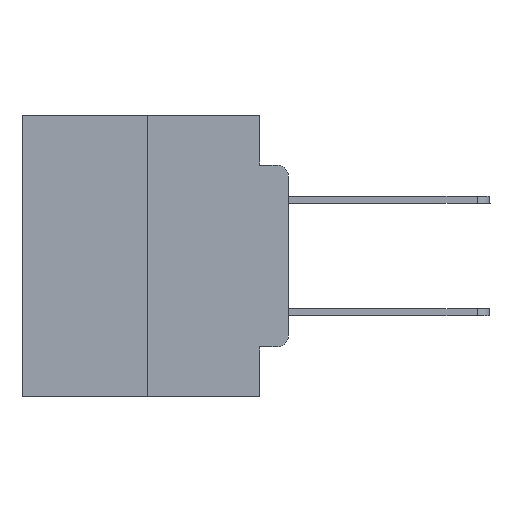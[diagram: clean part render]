
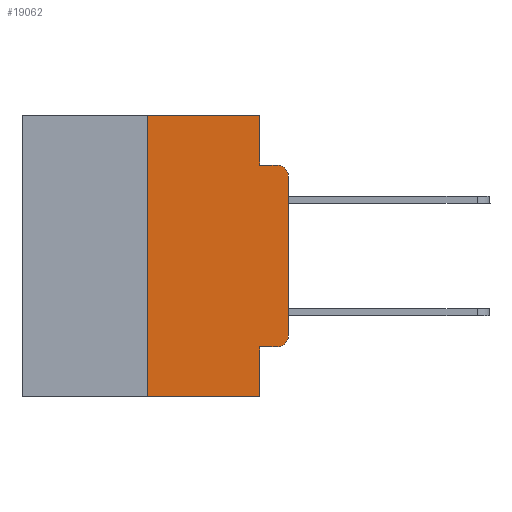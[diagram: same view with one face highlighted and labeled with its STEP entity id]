
A CAD part, left-side view. The second image highlights one B-rep face of the part: STEP entity #19062.
In plain terms, the highlighted planar face has unit normal (-1, 0, 0).
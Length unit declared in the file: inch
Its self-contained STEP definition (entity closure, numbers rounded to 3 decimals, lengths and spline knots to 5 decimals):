
#301 = DIRECTION ( 'NONE',  ( -1., 0., 0. ) ) ;
#646 = EDGE_CURVE ( 'NONE', #17560, #13822, #26466, .T. ) ;
#674 = VECTOR ( 'NONE', #2871, 39.37008 ) ;
#688 = CARTESIAN_POINT ( 'NONE',  ( 0., 0.051, 0. ) ) ;
#903 = CARTESIAN_POINT ( 'NONE',  ( 0., 0.051, -0.0885 ) ) ;
#1089 = VERTEX_POINT ( 'NONE', #4384 ) ;
#2356 = DIRECTION ( 'NONE',  ( 0., 0., -1. ) ) ;
#2700 = VERTEX_POINT ( 'NONE', #14157 ) ;
#2746 = ORIENTED_EDGE ( 'NONE', *, *, #14768, .T. ) ;
#2825 = DIRECTION ( 'NONE',  ( 0., 0., 1. ) ) ;
#2871 = DIRECTION ( 'NONE',  ( 0., -1., 0. ) ) ;
#2971 = EDGE_CURVE ( 'NONE', #7550, #22965, #7790, .T. ) ;
#3133 = EDGE_CURVE ( 'NONE', #5858, #2700, #3486, .T. ) ;
#3486 = CIRCLE ( 'NONE', #5319, 0.02 ) ;
#3711 = VECTOR ( 'NONE', #15448, 39.37008 ) ;
#4319 = VECTOR ( 'NONE', #15468, 39.37008 ) ;
#4364 = LINE ( 'NONE', #21749, #3711 ) ;
#4384 = CARTESIAN_POINT ( 'NONE',  ( 0., 0.051, -0.4115 ) ) ;
#4393 = CARTESIAN_POINT ( 'NONE',  ( 0., 0.02, -0.1085 ) ) ;
#4721 = VECTOR ( 'NONE', #10827, 39.37008 ) ;
#5225 = ORIENTED_EDGE ( 'NONE', *, *, #14411, .T. ) ;
#5319 = AXIS2_PLACEMENT_3D ( 'NONE', #8738, #301, #23548 ) ;
#5858 = VERTEX_POINT ( 'NONE', #16393 ) ;
#6036 = ORIENTED_EDGE ( 'NONE', *, *, #646, .F. ) ;
#6722 = LINE ( 'NONE', #23231, #4721 ) ;
#7337 = ORIENTED_EDGE ( 'NONE', *, *, #17486, .T. ) ;
#7550 = VERTEX_POINT ( 'NONE', #10167 ) ;
#7790 = CIRCLE ( 'NONE', #11848, 0.02 ) ;
#8301 = LINE ( 'NONE', #9455, #674 ) ;
#8578 = CARTESIAN_POINT ( 'NONE',  ( 0., 0.051, -0.5 ) ) ;
#8738 = CARTESIAN_POINT ( 'NONE',  ( 0., 0.02, -0.3915 ) ) ;
#8921 = EDGE_CURVE ( 'NONE', #1089, #23056, #6722, .T. ) ;
#9004 = CARTESIAN_POINT ( 'NONE',  ( 0., 0.051, 0. ) ) ;
#9455 = CARTESIAN_POINT ( 'NONE',  ( 0., 0.051, -0.4115 ) ) ;
#9891 = DIRECTION ( 'NONE',  ( 0., 0., -1. ) ) ;
#9920 = EDGE_CURVE ( 'NONE', #17055, #17560, #24547, .T. ) ;
#10167 = CARTESIAN_POINT ( 'NONE',  ( 0., 0., -0.1085 ) ) ;
#10489 = ORIENTED_EDGE ( 'NONE', *, *, #14326, .F. ) ;
#10553 = AXIS2_PLACEMENT_3D ( 'NONE', #26771, #22561, #9891 ) ;
#10827 = DIRECTION ( 'NONE',  ( 0., 0., -1. ) ) ;
#11048 = CARTESIAN_POINT ( 'NONE',  ( 0., 0.25, -0.5 ) ) ;
#11074 = CARTESIAN_POINT ( 'NONE',  ( 0., 0.25, 0. ) ) ;
#11191 = EDGE_CURVE ( 'NONE', #13822, #22965, #26733, .T. ) ;
#11541 = DIRECTION ( 'NONE',  ( 0., -1., 0. ) ) ;
#11777 = VECTOR ( 'NONE', #2825, 39.37008 ) ;
#11848 = AXIS2_PLACEMENT_3D ( 'NONE', #4393, #22735, #2356 ) ;
#12806 = ORIENTED_EDGE ( 'NONE', *, *, #11191, .F. ) ;
#13822 = VERTEX_POINT ( 'NONE', #20030 ) ;
#14157 = CARTESIAN_POINT ( 'NONE',  ( 0., 0., -0.3915 ) ) ;
#14244 = VECTOR ( 'NONE', #25434, 39.37008 ) ;
#14326 = EDGE_CURVE ( 'NONE', #21789, #17055, #4364, .T. ) ;
#14411 = EDGE_CURVE ( 'NONE', #21789, #23056, #23899, .T. ) ;
#14768 = EDGE_CURVE ( 'NONE', #1089, #5858, #8301, .T. ) ;
#15448 = DIRECTION ( 'NONE',  ( 0., 0., 1. ) ) ;
#15468 = DIRECTION ( 'NONE',  ( 0., -1., 0. ) ) ;
#15838 = VECTOR ( 'NONE', #11541, 39.37008 ) ;
#16393 = CARTESIAN_POINT ( 'NONE',  ( 0., 0.02, -0.4115 ) ) ;
#16419 = LINE ( 'NONE', #21790, #11777 ) ;
#17055 = VERTEX_POINT ( 'NONE', #11074 ) ;
#17389 = CARTESIAN_POINT ( 'NONE',  ( 0., 0.473, 0. ) ) ;
#17486 = EDGE_CURVE ( 'NONE', #2700, #7550, #16419, .T. ) ;
#17560 = VERTEX_POINT ( 'NONE', #688 ) ;
#17788 = EDGE_LOOP ( 'NONE', ( #7337, #21321, #12806, #6036, #21413, #10489, #5225, #20785, #2746, #17831 ) ) ;
#17831 = ORIENTED_EDGE ( 'NONE', *, *, #3133, .T. ) ;
#17990 = PLANE ( 'NONE',  #10553 ) ;
#19037 = CARTESIAN_POINT ( 'NONE',  ( 0., 0.473, -0.5 ) ) ;
#19062 = ADVANCED_FACE ( 'NONE', ( #24620 ), #17990, .F. ) ;
#19707 = DIRECTION ( 'NONE',  ( 0., 0., -1. ) ) ;
#20030 = CARTESIAN_POINT ( 'NONE',  ( 0., 0.051, -0.0885 ) ) ;
#20785 = ORIENTED_EDGE ( 'NONE', *, *, #8921, .F. ) ;
#21321 = ORIENTED_EDGE ( 'NONE', *, *, #2971, .T. ) ;
#21413 = ORIENTED_EDGE ( 'NONE', *, *, #9920, .F. ) ;
#21749 = CARTESIAN_POINT ( 'NONE',  ( 0., 0.25, 0. ) ) ;
#21789 = VERTEX_POINT ( 'NONE', #11048 ) ;
#21790 = CARTESIAN_POINT ( 'NONE',  ( 0., 0., 0. ) ) ;
#22561 = DIRECTION ( 'NONE',  ( 1., 0., 0. ) ) ;
#22735 = DIRECTION ( 'NONE',  ( -1., 0., 0. ) ) ;
#22857 = CARTESIAN_POINT ( 'NONE',  ( 0., 0.02, -0.0885 ) ) ;
#22965 = VERTEX_POINT ( 'NONE', #22857 ) ;
#23056 = VERTEX_POINT ( 'NONE', #8578 ) ;
#23231 = CARTESIAN_POINT ( 'NONE',  ( 0., 0.051, 0. ) ) ;
#23548 = DIRECTION ( 'NONE',  ( 0., 0., -1. ) ) ;
#23899 = LINE ( 'NONE', #19037, #14244 ) ;
#24517 = VECTOR ( 'NONE', #19707, 39.37008 ) ;
#24547 = LINE ( 'NONE', #17389, #4319 ) ;
#24620 = FACE_OUTER_BOUND ( 'NONE', #17788, .T. ) ;
#25434 = DIRECTION ( 'NONE',  ( 0., -1., 0. ) ) ;
#26466 = LINE ( 'NONE', #9004, #24517 ) ;
#26733 = LINE ( 'NONE', #903, #15838 ) ;
#26771 = CARTESIAN_POINT ( 'NONE',  ( 0., 0.473, 0. ) ) ;
